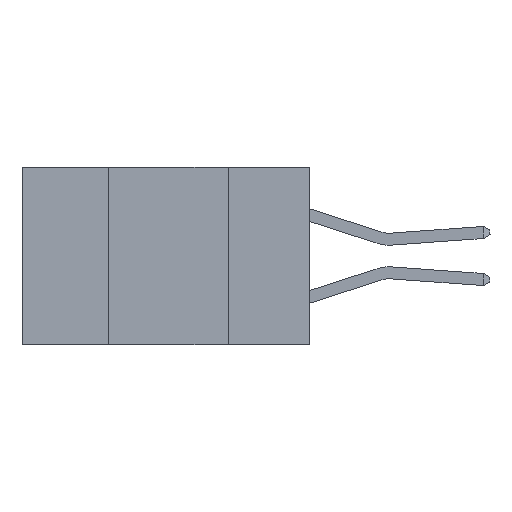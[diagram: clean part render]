
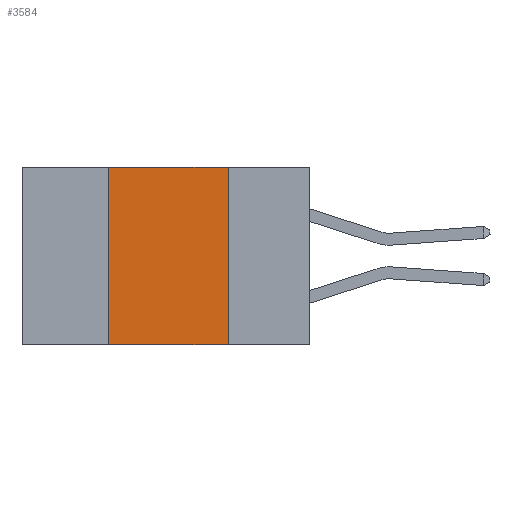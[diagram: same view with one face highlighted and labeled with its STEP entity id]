
A CAD part, left-side view. The second image highlights one B-rep face of the part: STEP entity #3584.
In plain terms, the highlighted planar face has unit normal (-1, 0, 0).
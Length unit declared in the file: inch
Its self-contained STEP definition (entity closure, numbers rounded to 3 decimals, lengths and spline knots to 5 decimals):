
#311 = EDGE_CURVE ( 'NONE', #6615, #6475, #9390, .T. ) ;
#376 = DIRECTION ( 'NONE',  ( 0., -1., 0. ) ) ;
#1524 = CARTESIAN_POINT ( 'NONE',  ( 0., 0.6, 0. ) ) ;
#1785 = ORIENTED_EDGE ( 'NONE', *, *, #3852, .T. ) ;
#2188 = CARTESIAN_POINT ( 'NONE',  ( 0., 0.17, 0. ) ) ;
#2191 = ORIENTED_EDGE ( 'NONE', *, *, #311, .F. ) ;
#2672 = PLANE ( 'NONE',  #11158 ) ;
#2976 = DIRECTION ( 'NONE',  ( 0., -1., 0. ) ) ;
#3101 = DIRECTION ( 'NONE',  ( 0., 0., -1. ) ) ;
#3584 = ADVANCED_FACE ( 'NONE', ( #7277 ), #2672, .F. ) ;
#3852 = EDGE_CURVE ( 'NONE', #7643, #6475, #12275, .T. ) ;
#3994 = EDGE_LOOP ( 'NONE', ( #2191, #9078, #10893, #1785 ) ) ;
#4126 = VERTEX_POINT ( 'NONE', #11788 ) ;
#4949 = DIRECTION ( 'NONE',  ( 1., 0., 0. ) ) ;
#5077 = EDGE_CURVE ( 'NONE', #4126, #6615, #12968, .T. ) ;
#5575 = VECTOR ( 'NONE', #3101, 39.37008 ) ;
#5806 = CARTESIAN_POINT ( 'NONE',  ( 0., 0.42, -0.37 ) ) ;
#6072 = VECTOR ( 'NONE', #2976, 39.37008 ) ;
#6475 = VERTEX_POINT ( 'NONE', #7239 ) ;
#6615 = VERTEX_POINT ( 'NONE', #2188 ) ;
#6821 = CARTESIAN_POINT ( 'NONE',  ( 0., 0.6, 0. ) ) ;
#6947 = CARTESIAN_POINT ( 'NONE',  ( 0., 0.42, -0.37 ) ) ;
#7181 = CARTESIAN_POINT ( 'NONE',  ( 0., 0.6, -0.37 ) ) ;
#7239 = CARTESIAN_POINT ( 'NONE',  ( 0., 0.17, -0.37 ) ) ;
#7277 = FACE_OUTER_BOUND ( 'NONE', #3994, .T. ) ;
#7643 = VERTEX_POINT ( 'NONE', #6947 ) ;
#8728 = VECTOR ( 'NONE', #13091, 39.37008 ) ;
#9078 = ORIENTED_EDGE ( 'NONE', *, *, #5077, .F. ) ;
#9390 = LINE ( 'NONE', #12342, #5575 ) ;
#9922 = VECTOR ( 'NONE', #376, 39.37008 ) ;
#10039 = LINE ( 'NONE', #5806, #8728 ) ;
#10532 = EDGE_CURVE ( 'NONE', #7643, #4126, #10039, .T. ) ;
#10893 = ORIENTED_EDGE ( 'NONE', *, *, #10532, .F. ) ;
#10909 = DIRECTION ( 'NONE',  ( 0., 0., -1. ) ) ;
#11158 = AXIS2_PLACEMENT_3D ( 'NONE', #6821, #4949, #10909 ) ;
#11788 = CARTESIAN_POINT ( 'NONE',  ( 0., 0.42, 0. ) ) ;
#12275 = LINE ( 'NONE', #7181, #6072 ) ;
#12342 = CARTESIAN_POINT ( 'NONE',  ( 0., 0.17, -0.37 ) ) ;
#12968 = LINE ( 'NONE', #1524, #9922 ) ;
#13091 = DIRECTION ( 'NONE',  ( 0., 0., 1. ) ) ;
